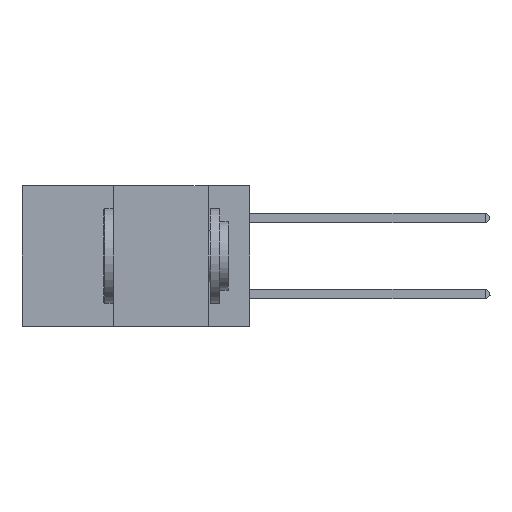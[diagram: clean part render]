
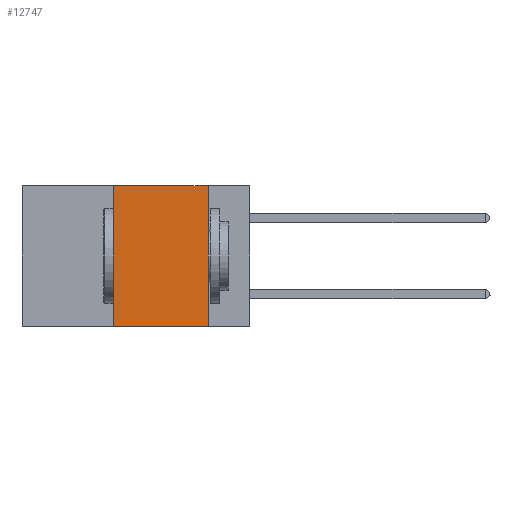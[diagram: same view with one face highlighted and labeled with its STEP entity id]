
A CAD part, left-side view. The second image highlights one B-rep face of the part: STEP entity #12747.
In plain terms, the highlighted planar face has unit normal (-1, 0, 0).
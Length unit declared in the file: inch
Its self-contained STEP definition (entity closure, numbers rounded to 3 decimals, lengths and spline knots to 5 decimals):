
#128 = FACE_OUTER_BOUND ( 'NONE', #34861, .T. ) ;
#2592 = CARTESIAN_POINT ( 'NONE',  ( 0., 0.6, 0. ) ) ;
#3302 = CARTESIAN_POINT ( 'NONE',  ( 0., 0.6, -0.37 ) ) ;
#5214 = VECTOR ( 'NONE', #28282, 39.37008 ) ;
#6706 = AXIS2_PLACEMENT_3D ( 'NONE', #2592, #6785, #9027 ) ;
#6756 = CARTESIAN_POINT ( 'NONE',  ( 0., 0.11, 0. ) ) ;
#6785 = DIRECTION ( 'NONE',  ( 1., 0., 0. ) ) ;
#7023 = DIRECTION ( 'NONE',  ( 0., 0., -1. ) ) ;
#7671 = VECTOR ( 'NONE', #32483, 39.37008 ) ;
#8566 = EDGE_CURVE ( 'NONE', #24348, #27779, #28414, .T. ) ;
#9027 = DIRECTION ( 'NONE',  ( 0., 0., -1. ) ) ;
#9681 = CARTESIAN_POINT ( 'NONE',  ( 0., 0.6, 0. ) ) ;
#10194 = ORIENTED_EDGE ( 'NONE', *, *, #26805, .F. ) ;
#11547 = CARTESIAN_POINT ( 'NONE',  ( 0., 0.11, 0. ) ) ;
#12747 = ADVANCED_FACE ( 'NONE', ( #128 ), #14956, .F. ) ;
#14956 = PLANE ( 'NONE',  #6706 ) ;
#15181 = ORIENTED_EDGE ( 'NONE', *, *, #19101, .F. ) ;
#17984 = VECTOR ( 'NONE', #39946, 39.37008 ) ;
#19101 = EDGE_CURVE ( 'NONE', #27779, #23258, #34881, .T. ) ;
#20343 = EDGE_CURVE ( 'NONE', #24348, #27093, #34325, .T. ) ;
#23258 = VERTEX_POINT ( 'NONE', #11547 ) ;
#24348 = VERTEX_POINT ( 'NONE', #26193 ) ;
#26193 = CARTESIAN_POINT ( 'NONE',  ( 0., 0.36, -0.37 ) ) ;
#26441 = CARTESIAN_POINT ( 'NONE',  ( 0., 0.36, 0. ) ) ;
#26805 = EDGE_CURVE ( 'NONE', #23258, #27093, #29332, .T. ) ;
#27093 = VERTEX_POINT ( 'NONE', #28817 ) ;
#27779 = VERTEX_POINT ( 'NONE', #26441 ) ;
#27888 = ORIENTED_EDGE ( 'NONE', *, *, #20343, .T. ) ;
#28282 = DIRECTION ( 'NONE',  ( 0., -1., 0. ) ) ;
#28367 = VECTOR ( 'NONE', #7023, 39.37008 ) ;
#28414 = LINE ( 'NONE', #39535, #17984 ) ;
#28817 = CARTESIAN_POINT ( 'NONE',  ( 0., 0.11, -0.37 ) ) ;
#29332 = LINE ( 'NONE', #6756, #28367 ) ;
#32434 = ORIENTED_EDGE ( 'NONE', *, *, #8566, .F. ) ;
#32483 = DIRECTION ( 'NONE',  ( 0., -1., 0. ) ) ;
#34325 = LINE ( 'NONE', #3302, #7671 ) ;
#34861 = EDGE_LOOP ( 'NONE', ( #10194, #15181, #32434, #27888 ) ) ;
#34881 = LINE ( 'NONE', #9681, #5214 ) ;
#39535 = CARTESIAN_POINT ( 'NONE',  ( 0., 0.36, 0. ) ) ;
#39946 = DIRECTION ( 'NONE',  ( 0., 0., 1. ) ) ;
